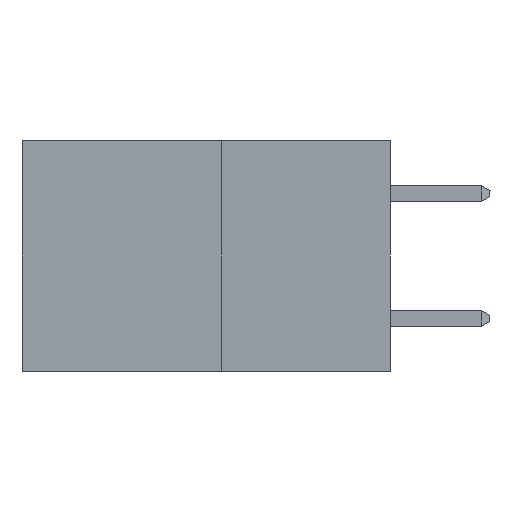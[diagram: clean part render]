
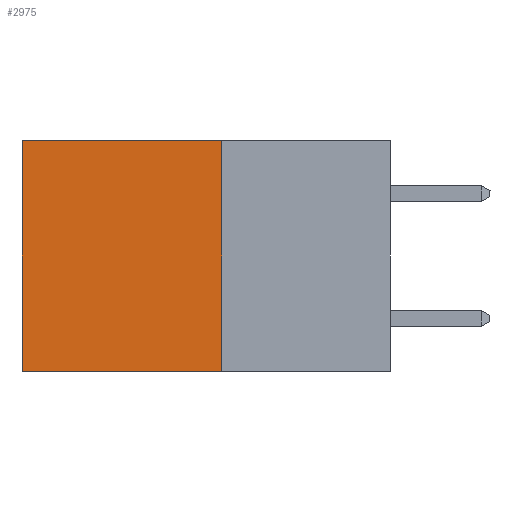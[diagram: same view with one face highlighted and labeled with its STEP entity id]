
A CAD part, left-side view. The second image highlights one B-rep face of the part: STEP entity #2975.
In plain terms, the highlighted planar face has unit normal (-1, 0, 0).
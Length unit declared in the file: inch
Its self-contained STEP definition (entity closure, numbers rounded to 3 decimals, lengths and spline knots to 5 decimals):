
#761 = DIRECTION ( 'NONE',  ( 0., 0., -1. ) ) ;
#1041 = EDGE_CURVE ( 'NONE', #7043, #7730, #3998, .T. ) ;
#1270 = CARTESIAN_POINT ( 'NONE',  ( 0.277, 0.27, 0. ) ) ;
#1440 = LINE ( 'NONE', #3377, #3875 ) ;
#2392 = CARTESIAN_POINT ( 'NONE',  ( 0.277, 0.27, -0.37 ) ) ;
#2975 = ADVANCED_FACE ( 'NONE', ( #8263 ), #3666, .F. ) ;
#3013 = VECTOR ( 'NONE', #761, 39.37008 ) ;
#3339 = CARTESIAN_POINT ( 'NONE',  ( 0.277, 0.59, 0. ) ) ;
#3377 = CARTESIAN_POINT ( 'NONE',  ( 0.277, 0.27, -0.37 ) ) ;
#3497 = VECTOR ( 'NONE', #7993, 39.37008 ) ;
#3576 = CARTESIAN_POINT ( 'NONE',  ( 0.277, 0.27, -0.37 ) ) ;
#3666 = PLANE ( 'NONE',  #10479 ) ;
#3875 = VECTOR ( 'NONE', #4288, 39.37008 ) ;
#3902 = CARTESIAN_POINT ( 'NONE',  ( 0.277, 0.27, -0.37 ) ) ;
#3998 = LINE ( 'NONE', #10636, #8464 ) ;
#4288 = DIRECTION ( 'NONE',  ( 0., 1., 0. ) ) ;
#4965 = LINE ( 'NONE', #3902, #3013 ) ;
#5394 = CARTESIAN_POINT ( 'NONE',  ( 0.277, 0.59, -0.37 ) ) ;
#5450 = EDGE_CURVE ( 'NONE', #10416, #7730, #1440, .T. ) ;
#5974 = LINE ( 'NONE', #11333, #3497 ) ;
#7043 = VERTEX_POINT ( 'NONE', #3339 ) ;
#7730 = VERTEX_POINT ( 'NONE', #5394 ) ;
#7942 = DIRECTION ( 'NONE',  ( 0., 0., -1. ) ) ;
#7993 = DIRECTION ( 'NONE',  ( 0., 1., 0. ) ) ;
#8021 = DIRECTION ( 'NONE',  ( 1., 0., 0. ) ) ;
#8263 = FACE_OUTER_BOUND ( 'NONE', #11664, .T. ) ;
#8397 = VERTEX_POINT ( 'NONE', #1270 ) ;
#8440 = EDGE_CURVE ( 'NONE', #8397, #7043, #5974, .T. ) ;
#8464 = VECTOR ( 'NONE', #11546, 39.37008 ) ;
#8891 = EDGE_CURVE ( 'NONE', #8397, #10416, #4965, .T. ) ;
#8965 = ORIENTED_EDGE ( 'NONE', *, *, #5450, .F. ) ;
#9758 = ORIENTED_EDGE ( 'NONE', *, *, #1041, .T. ) ;
#10416 = VERTEX_POINT ( 'NONE', #2392 ) ;
#10479 = AXIS2_PLACEMENT_3D ( 'NONE', #3576, #8021, #7942 ) ;
#10636 = CARTESIAN_POINT ( 'NONE',  ( 0.277, 0.59, -0.37 ) ) ;
#10915 = ORIENTED_EDGE ( 'NONE', *, *, #8440, .T. ) ;
#11169 = ORIENTED_EDGE ( 'NONE', *, *, #8891, .F. ) ;
#11333 = CARTESIAN_POINT ( 'NONE',  ( 0.277, 0.27, 0. ) ) ;
#11546 = DIRECTION ( 'NONE',  ( 0., 0., -1. ) ) ;
#11664 = EDGE_LOOP ( 'NONE', ( #9758, #8965, #11169, #10915 ) ) ;
